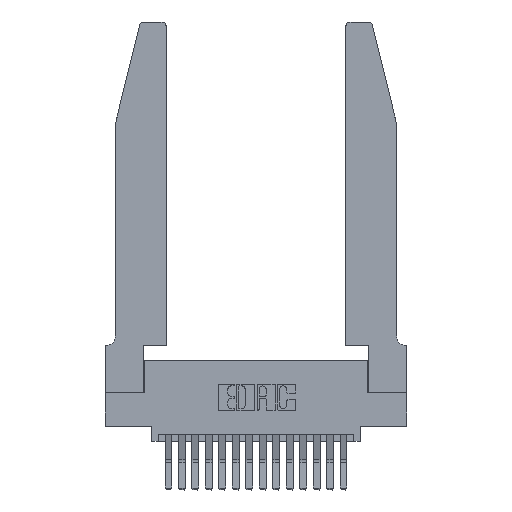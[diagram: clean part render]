
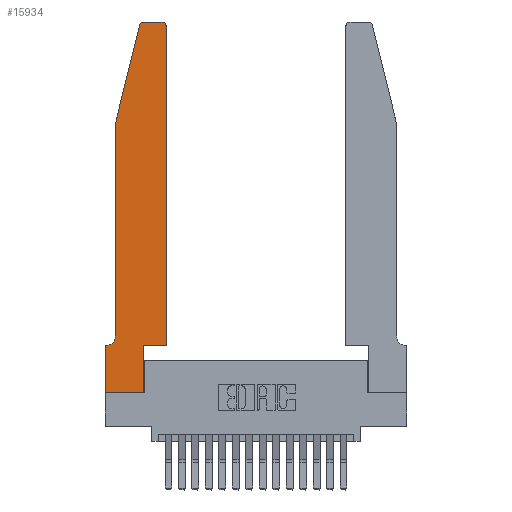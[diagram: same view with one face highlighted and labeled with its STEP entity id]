
A CAD part, top view. The second image highlights one B-rep face of the part: STEP entity #15934.
In plain terms, the highlighted planar face has unit normal (0, 0, 1).
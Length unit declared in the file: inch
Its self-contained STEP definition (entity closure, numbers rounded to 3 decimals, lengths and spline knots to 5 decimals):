
#47 = VERTEX_POINT ( 'NONE', #17968 ) ;
#580 = EDGE_LOOP ( 'NONE', ( #18090, #12345, #12236, #19234, #8268, #10291, #7956, #19441, #19076, #3710, #2470, #15723 ) ) ;
#606 = CARTESIAN_POINT ( 'NONE',  ( 0., 0.35, 0.37 ) ) ;
#608 = CARTESIAN_POINT ( 'NONE',  ( 0.0755, 2., 0.37 ) ) ;
#810 = EDGE_CURVE ( 'NONE', #10678, #6154, #6606, .T. ) ;
#996 = CARTESIAN_POINT ( 'NONE',  ( 0.4505, 2.72, 0.37 ) ) ;
#1229 = AXIS2_PLACEMENT_3D ( 'NONE', #15195, #6204, #16719 ) ;
#2169 = DIRECTION ( 'NONE',  ( 0., 0., 1. ) ) ;
#2344 = VECTOR ( 'NONE', #16343, 39.37008 ) ;
#2367 = VECTOR ( 'NONE', #18427, 39.37008 ) ;
#2470 = ORIENTED_EDGE ( 'NONE', *, *, #8993, .T. ) ;
#2502 = EDGE_CURVE ( 'NONE', #8559, #8490, #8250, .T. ) ;
#2528 = CARTESIAN_POINT ( 'NONE',  ( 0.4505, 0.35, 0.37 ) ) ;
#2626 = CARTESIAN_POINT ( 'NONE',  ( 0.2605, 2.75, 0.37 ) ) ;
#3005 = EDGE_CURVE ( 'NONE', #11682, #16421, #9015, .T. ) ;
#3710 = ORIENTED_EDGE ( 'NONE', *, *, #8616, .T. ) ;
#3856 = VERTEX_POINT ( 'NONE', #996 ) ;
#3900 = EDGE_CURVE ( 'NONE', #7207, #13592, #15207, .T. ) ;
#4321 = VECTOR ( 'NONE', #12981, 39.37008 ) ;
#4390 = LINE ( 'NONE', #10742, #16497 ) ;
#4551 = VECTOR ( 'NONE', #6301, 39.37008 ) ;
#4642 = DIRECTION ( 'NONE',  ( 0., 0., -1. ) ) ;
#4884 = AXIS2_PLACEMENT_3D ( 'NONE', #13762, #4642, #15235 ) ;
#4937 = DIRECTION ( 'NONE',  ( 0., 1., 0. ) ) ;
#5008 = CARTESIAN_POINT ( 'NONE',  ( 0., 0., 0.37 ) ) ;
#5227 = LINE ( 'NONE', #608, #12868 ) ;
#5244 = CARTESIAN_POINT ( 'NONE',  ( 0.0755, 2., 0.37 ) ) ;
#5310 = VERTEX_POINT ( 'NONE', #19734 ) ;
#6154 = VERTEX_POINT ( 'NONE', #14979 ) ;
#6204 = DIRECTION ( 'NONE',  ( 0., 0., 1. ) ) ;
#6235 = CARTESIAN_POINT ( 'NONE',  ( 0.0755, 0.35, 0.37 ) ) ;
#6259 = AXIS2_PLACEMENT_3D ( 'NONE', #10049, #2169, #12979 ) ;
#6301 = DIRECTION ( 'NONE',  ( -1., 0., 0. ) ) ;
#6606 = LINE ( 'NONE', #14333, #2367 ) ;
#7207 = VERTEX_POINT ( 'NONE', #8453 ) ;
#7467 = DIRECTION ( 'NONE',  ( 0., 0., 1. ) ) ;
#7498 = FACE_OUTER_BOUND ( 'NONE', #580, .T. ) ;
#7550 = EDGE_CURVE ( 'NONE', #8490, #10678, #4390, .T. ) ;
#7689 = CARTESIAN_POINT ( 'NONE',  ( 0.4205, 2.75, 0.37 ) ) ;
#7956 = ORIENTED_EDGE ( 'NONE', *, *, #7550, .T. ) ;
#8106 = CARTESIAN_POINT ( 'NONE',  ( 0.0755, 0.42, 0.37 ) ) ;
#8250 = LINE ( 'NONE', #6235, #4551 ) ;
#8268 = ORIENTED_EDGE ( 'NONE', *, *, #12685, .T. ) ;
#8453 = CARTESIAN_POINT ( 'NONE',  ( 0.284, 2.75, 0.37 ) ) ;
#8490 = VERTEX_POINT ( 'NONE', #606 ) ;
#8524 = VECTOR ( 'NONE', #4937, 39.37008 ) ;
#8559 = VERTEX_POINT ( 'NONE', #17629 ) ;
#8616 = EDGE_CURVE ( 'NONE', #47, #5310, #14584, .T. ) ;
#8875 = VERTEX_POINT ( 'NONE', #7689 ) ;
#8993 = EDGE_CURVE ( 'NONE', #5310, #3856, #16437, .T. ) ;
#9015 = LINE ( 'NONE', #5244, #4321 ) ;
#9704 = DIRECTION ( 'NONE',  ( 0., 1., 0. ) ) ;
#9840 = CIRCLE ( 'NONE', #4884, 0.07 ) ;
#10049 = CARTESIAN_POINT ( 'NONE',  ( 0., 0.35, 0.37 ) ) ;
#10291 = ORIENTED_EDGE ( 'NONE', *, *, #2502, .T. ) ;
#10476 = EDGE_CURVE ( 'NONE', #3856, #8875, #15920, .T. ) ;
#10678 = VERTEX_POINT ( 'NONE', #5008 ) ;
#10742 = CARTESIAN_POINT ( 'NONE',  ( 0., 0., 0.37 ) ) ;
#11614 = DIRECTION ( 'NONE',  ( -0.239, -0.971, 0. ) ) ;
#11682 = VERTEX_POINT ( 'NONE', #14253 ) ;
#12236 = ORIENTED_EDGE ( 'NONE', *, *, #17742, .T. ) ;
#12345 = ORIENTED_EDGE ( 'NONE', *, *, #3900, .T. ) ;
#12438 = VECTOR ( 'NONE', #14983, 39.37008 ) ;
#12576 = CARTESIAN_POINT ( 'NONE',  ( 0.4505, 0.35, 0.37 ) ) ;
#12685 = EDGE_CURVE ( 'NONE', #16421, #8559, #9840, .T. ) ;
#12868 = VECTOR ( 'NONE', #11614, 39.37008 ) ;
#12979 = DIRECTION ( 'NONE',  ( 1., 0., 0. ) ) ;
#12981 = DIRECTION ( 'NONE',  ( 0., -1., 0. ) ) ;
#13592 = VERTEX_POINT ( 'NONE', #14633 ) ;
#13762 = CARTESIAN_POINT ( 'NONE',  ( 0.0055, 0.42, 0.37 ) ) ;
#14253 = CARTESIAN_POINT ( 'NONE',  ( 0.0755, 2., 0.37 ) ) ;
#14333 = CARTESIAN_POINT ( 'NONE',  ( 0., 0., 0.37 ) ) ;
#14584 = LINE ( 'NONE', #2528, #2344 ) ;
#14633 = CARTESIAN_POINT ( 'NONE',  ( 0.25487, 2.72718, 0.37 ) ) ;
#14690 = VECTOR ( 'NONE', #9704, 39.37008 ) ;
#14979 = CARTESIAN_POINT ( 'NONE',  ( 0.2865, 0., 0.37 ) ) ;
#14983 = DIRECTION ( 'NONE',  ( -1., 0., 0. ) ) ;
#15195 = CARTESIAN_POINT ( 'NONE',  ( 0.4205, 2.72, 0.37 ) ) ;
#15207 = CIRCLE ( 'NONE', #19015, 0.03 ) ;
#15235 = DIRECTION ( 'NONE',  ( -1., 0., 0. ) ) ;
#15723 = ORIENTED_EDGE ( 'NONE', *, *, #10476, .T. ) ;
#15920 = CIRCLE ( 'NONE', #1229, 0.03 ) ;
#15934 = ADVANCED_FACE ( 'NONE', ( #7498 ), #18833, .T. ) ;
#16343 = DIRECTION ( 'NONE',  ( 1., 0., 0. ) ) ;
#16354 = LINE ( 'NONE', #2626, #12438 ) ;
#16421 = VERTEX_POINT ( 'NONE', #8106 ) ;
#16437 = LINE ( 'NONE', #12576, #8524 ) ;
#16447 = CARTESIAN_POINT ( 'NONE',  ( 0.284, 2.72, 0.37 ) ) ;
#16497 = VECTOR ( 'NONE', #19471, 39.37008 ) ;
#16719 = DIRECTION ( 'NONE',  ( 1., 0., 0. ) ) ;
#17037 = CARTESIAN_POINT ( 'NONE',  ( 0.2865, 0.35, 0.37 ) ) ;
#17313 = EDGE_CURVE ( 'NONE', #8875, #7207, #16354, .T. ) ;
#17629 = CARTESIAN_POINT ( 'NONE',  ( 0.0055, 0.35, 0.37 ) ) ;
#17742 = EDGE_CURVE ( 'NONE', #13592, #11682, #5227, .T. ) ;
#17940 = DIRECTION ( 'NONE',  ( 1., 0., 0. ) ) ;
#17968 = CARTESIAN_POINT ( 'NONE',  ( 0.2865, 0.35, 0.37 ) ) ;
#18090 = ORIENTED_EDGE ( 'NONE', *, *, #17313, .T. ) ;
#18106 = EDGE_CURVE ( 'NONE', #6154, #47, #18611, .T. ) ;
#18427 = DIRECTION ( 'NONE',  ( 1., 0., 0. ) ) ;
#18611 = LINE ( 'NONE', #17037, #14690 ) ;
#18833 = PLANE ( 'NONE',  #6259 ) ;
#19015 = AXIS2_PLACEMENT_3D ( 'NONE', #16447, #7467, #17940 ) ;
#19076 = ORIENTED_EDGE ( 'NONE', *, *, #18106, .T. ) ;
#19234 = ORIENTED_EDGE ( 'NONE', *, *, #3005, .T. ) ;
#19441 = ORIENTED_EDGE ( 'NONE', *, *, #810, .T. ) ;
#19471 = DIRECTION ( 'NONE',  ( 0., -1., 0. ) ) ;
#19734 = CARTESIAN_POINT ( 'NONE',  ( 0.4505, 0.35, 0.37 ) ) ;
